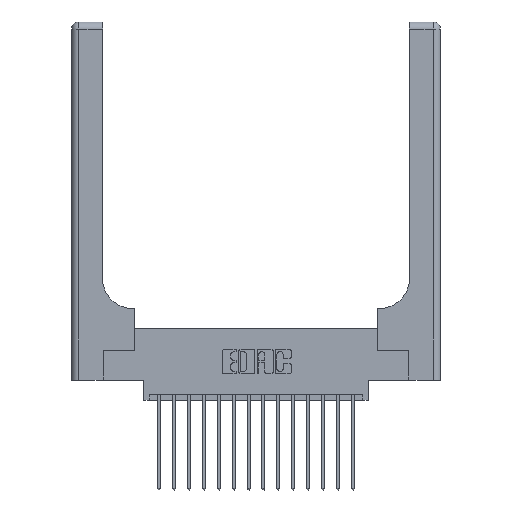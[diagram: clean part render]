
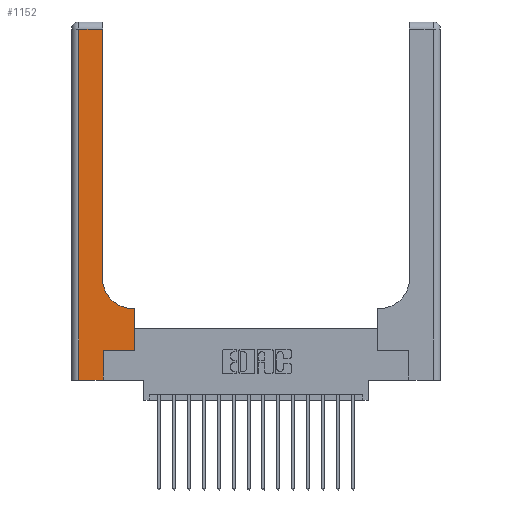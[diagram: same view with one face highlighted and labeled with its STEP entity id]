
A CAD part, top view. The second image highlights one B-rep face of the part: STEP entity #1152.
In plain terms, the highlighted planar face has unit normal (0, 0, 1).
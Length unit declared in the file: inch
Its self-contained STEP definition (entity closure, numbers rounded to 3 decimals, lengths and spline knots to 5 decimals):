
#143 = CARTESIAN_POINT ( 'NONE',  ( 0.265, 0.25, 0.37 ) ) ;
#348 = DIRECTION ( 'NONE',  ( 0., 0., -1. ) ) ;
#860 = ORIENTED_EDGE ( 'NONE', *, *, #6096, .T. ) ;
#1152 = ADVANCED_FACE ( 'NONE', ( #3287 ), #17490, .F. ) ;
#1286 = AXIS2_PLACEMENT_3D ( 'NONE', #2765, #14197, #13814 ) ;
#1463 = LINE ( 'NONE', #5877, #1867 ) ;
#1540 = EDGE_LOOP ( 'NONE', ( #13471, #12471, #2438, #17955, #860, #15712, #17799, #6995, #3562 ) ) ;
#1644 = VERTEX_POINT ( 'NONE', #7036 ) ;
#1782 = DIRECTION ( 'NONE',  ( 1., 0., 0. ) ) ;
#1867 = VECTOR ( 'NONE', #11669, 39.37008 ) ;
#1899 = VECTOR ( 'NONE', #11689, 39.37008 ) ;
#2012 = LINE ( 'NONE', #7777, #12959 ) ;
#2360 = VECTOR ( 'NONE', #13304, 39.37008 ) ;
#2438 = ORIENTED_EDGE ( 'NONE', *, *, #6067, .T. ) ;
#2491 = VERTEX_POINT ( 'NONE', #12869 ) ;
#2765 = CARTESIAN_POINT ( 'NONE',  ( 0.51, 0.85, 0.37 ) ) ;
#3104 = CARTESIAN_POINT ( 'NONE',  ( 0., 3., 0.37 ) ) ;
#3287 = FACE_OUTER_BOUND ( 'NONE', #1540, .T. ) ;
#3562 = ORIENTED_EDGE ( 'NONE', *, *, #13311, .T. ) ;
#3844 = CARTESIAN_POINT ( 'NONE',  ( 0.528, 0.6, 0.37 ) ) ;
#4003 = CARTESIAN_POINT ( 'NONE',  ( 0.26, 3., 0.37 ) ) ;
#4684 = CARTESIAN_POINT ( 'NONE',  ( 0.265, 0., 0.37 ) ) ;
#4874 = EDGE_CURVE ( 'NONE', #8838, #12628, #1463, .T. ) ;
#5574 = EDGE_CURVE ( 'NONE', #1644, #13920, #11165, .T. ) ;
#5703 = LINE ( 'NONE', #12934, #17024 ) ;
#5817 = EDGE_CURVE ( 'NONE', #12558, #2491, #11243, .T. ) ;
#5877 = CARTESIAN_POINT ( 'NONE',  ( 0.528, 0.25, 0.37 ) ) ;
#6032 = VECTOR ( 'NONE', #13816, 39.37008 ) ;
#6067 = EDGE_CURVE ( 'NONE', #11405, #12558, #5703, .T. ) ;
#6096 = EDGE_CURVE ( 'NONE', #2491, #6714, #9295, .T. ) ;
#6097 = VERTEX_POINT ( 'NONE', #10256 ) ;
#6108 = DIRECTION ( 'NONE',  ( -1., 0., 0. ) ) ;
#6322 = DIRECTION ( 'NONE',  ( -1., 0., 0. ) ) ;
#6413 = CARTESIAN_POINT ( 'NONE',  ( 0.26, 0.6, 0.37 ) ) ;
#6714 = VERTEX_POINT ( 'NONE', #143 ) ;
#6888 = VECTOR ( 'NONE', #6322, 39.37008 ) ;
#6995 = ORIENTED_EDGE ( 'NONE', *, *, #8086, .T. ) ;
#7036 = CARTESIAN_POINT ( 'NONE',  ( 0.26, 0.85, 0.37 ) ) ;
#7777 = CARTESIAN_POINT ( 'NONE',  ( 0., 2.94, 0.37 ) ) ;
#8086 = EDGE_CURVE ( 'NONE', #12628, #6097, #15426, .T. ) ;
#8371 = EDGE_CURVE ( 'NONE', #6714, #8838, #10354, .T. ) ;
#8838 = VERTEX_POINT ( 'NONE', #16418 ) ;
#8952 = CARTESIAN_POINT ( 'NONE',  ( 0.265, 0.25, 0.37 ) ) ;
#9247 = CARTESIAN_POINT ( 'NONE',  ( 0., 0., 0.37 ) ) ;
#9295 = LINE ( 'NONE', #4684, #1899 ) ;
#9412 = EDGE_CURVE ( 'NONE', #13920, #11405, #2012, .T. ) ;
#10256 = CARTESIAN_POINT ( 'NONE',  ( 0.51, 0.6, 0.37 ) ) ;
#10354 = LINE ( 'NONE', #8952, #2360 ) ;
#11165 = LINE ( 'NONE', #4003, #6032 ) ;
#11243 = LINE ( 'NONE', #9247, #14769 ) ;
#11405 = VERTEX_POINT ( 'NONE', #17864 ) ;
#11669 = DIRECTION ( 'NONE',  ( 0., 1., 0. ) ) ;
#11689 = DIRECTION ( 'NONE',  ( 0., 1., 0. ) ) ;
#11982 = AXIS2_PLACEMENT_3D ( 'NONE', #3104, #348, #6108 ) ;
#12075 = CARTESIAN_POINT ( 'NONE',  ( 0.26, 2.94, 0.37 ) ) ;
#12471 = ORIENTED_EDGE ( 'NONE', *, *, #9412, .T. ) ;
#12558 = VERTEX_POINT ( 'NONE', #18052 ) ;
#12628 = VERTEX_POINT ( 'NONE', #3844 ) ;
#12869 = CARTESIAN_POINT ( 'NONE',  ( 0.265, 0., 0.37 ) ) ;
#12934 = CARTESIAN_POINT ( 'NONE',  ( 0.06, 3., 0.37 ) ) ;
#12959 = VECTOR ( 'NONE', #17924, 39.37008 ) ;
#13304 = DIRECTION ( 'NONE',  ( 1., 0., 0. ) ) ;
#13311 = EDGE_CURVE ( 'NONE', #6097, #1644, #17912, .T. ) ;
#13471 = ORIENTED_EDGE ( 'NONE', *, *, #5574, .T. ) ;
#13814 = DIRECTION ( 'NONE',  ( 1., 0., 0. ) ) ;
#13816 = DIRECTION ( 'NONE',  ( 0., 1., 0. ) ) ;
#13920 = VERTEX_POINT ( 'NONE', #12075 ) ;
#14197 = DIRECTION ( 'NONE',  ( 0., 0., -1. ) ) ;
#14769 = VECTOR ( 'NONE', #1782, 39.37008 ) ;
#15426 = LINE ( 'NONE', #6413, #6888 ) ;
#15712 = ORIENTED_EDGE ( 'NONE', *, *, #8371, .T. ) ;
#16418 = CARTESIAN_POINT ( 'NONE',  ( 0.528, 0.25, 0.37 ) ) ;
#17024 = VECTOR ( 'NONE', #17286, 39.37008 ) ;
#17286 = DIRECTION ( 'NONE',  ( 0., -1., 0. ) ) ;
#17490 = PLANE ( 'NONE',  #11982 ) ;
#17799 = ORIENTED_EDGE ( 'NONE', *, *, #4874, .T. ) ;
#17864 = CARTESIAN_POINT ( 'NONE',  ( 0.06, 2.94, 0.37 ) ) ;
#17912 = CIRCLE ( 'NONE', #1286, 0.25 ) ;
#17924 = DIRECTION ( 'NONE',  ( -1., 0., 0. ) ) ;
#17955 = ORIENTED_EDGE ( 'NONE', *, *, #5817, .T. ) ;
#18052 = CARTESIAN_POINT ( 'NONE',  ( 0.06, 0., 0.37 ) ) ;
